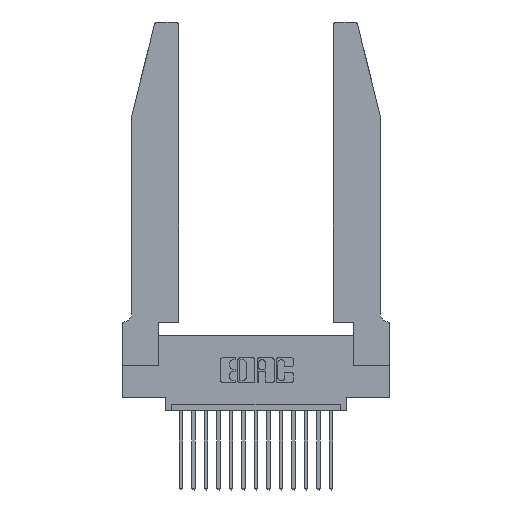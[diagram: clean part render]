
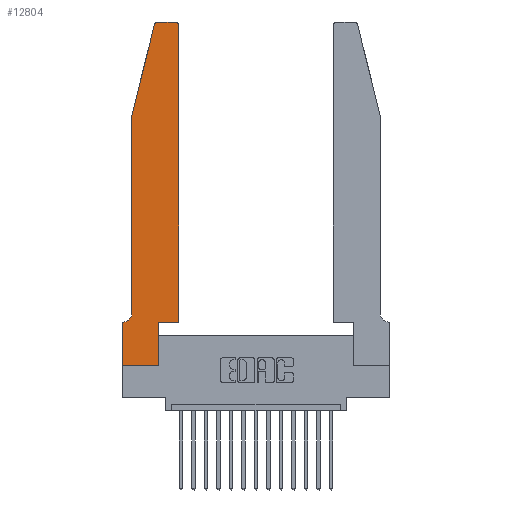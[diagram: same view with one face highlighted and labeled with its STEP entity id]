
A CAD part, top view. The second image highlights one B-rep face of the part: STEP entity #12804.
In plain terms, the highlighted planar face has unit normal (0, 0, 1).
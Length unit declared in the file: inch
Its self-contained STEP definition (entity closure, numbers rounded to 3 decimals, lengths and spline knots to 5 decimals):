
#98 = VECTOR ( 'NONE', #12148, 39.37008 ) ;
#214 = EDGE_CURVE ( 'NONE', #18326, #15537, #3929, .T. ) ;
#278 = VECTOR ( 'NONE', #9885, 39.37008 ) ;
#992 = CARTESIAN_POINT ( 'NONE',  ( 0.4505, 0.35, 0.37 ) ) ;
#1054 = VERTEX_POINT ( 'NONE', #13130 ) ;
#1116 = DIRECTION ( 'NONE',  ( 1., 0., 0. ) ) ;
#1184 = DIRECTION ( 'NONE',  ( 0., 0., -1. ) ) ;
#1329 = LINE ( 'NONE', #18397, #10377 ) ;
#1780 = ORIENTED_EDGE ( 'NONE', *, *, #1975, .T. ) ;
#1890 = AXIS2_PLACEMENT_3D ( 'NONE', #17011, #1184, #10670 ) ;
#1975 = EDGE_CURVE ( 'NONE', #15537, #5987, #3464, .T. ) ;
#1980 = DIRECTION ( 'NONE',  ( 1., 0., 0. ) ) ;
#1981 = VERTEX_POINT ( 'NONE', #3384 ) ;
#2617 = VERTEX_POINT ( 'NONE', #7955 ) ;
#2734 = EDGE_CURVE ( 'NONE', #1981, #7462, #11979, .T. ) ;
#3241 = CARTESIAN_POINT ( 'NONE',  ( 0.2605, 2.75, 0.37 ) ) ;
#3384 = CARTESIAN_POINT ( 'NONE',  ( 0.284, 2.75, 0.37 ) ) ;
#3448 = CARTESIAN_POINT ( 'NONE',  ( 0.2865, 0., 0.37 ) ) ;
#3463 = VERTEX_POINT ( 'NONE', #18270 ) ;
#3464 = LINE ( 'NONE', #7441, #11129 ) ;
#3508 = EDGE_LOOP ( 'NONE', ( #17701, #14174, #8043, #7591, #17520, #9115, #18115, #8007, #11388, #1780, #12761, #15362 ) ) ;
#3929 = LINE ( 'NONE', #10713, #98 ) ;
#4223 = DIRECTION ( 'NONE',  ( 1., 0., 0. ) ) ;
#4248 = VECTOR ( 'NONE', #13161, 39.37008 ) ;
#4614 = EDGE_CURVE ( 'NONE', #11953, #18326, #1329, .T. ) ;
#4631 = CARTESIAN_POINT ( 'NONE',  ( 0.0755, 2., 0.37 ) ) ;
#5124 = VECTOR ( 'NONE', #17776, 39.37008 ) ;
#5360 = CARTESIAN_POINT ( 'NONE',  ( 0.0755, 2., 0.37 ) ) ;
#5379 = DIRECTION ( 'NONE',  ( 0., 1., 0. ) ) ;
#5501 = DIRECTION ( 'NONE',  ( 0., 0., 1. ) ) ;
#5647 = CARTESIAN_POINT ( 'NONE',  ( 0.2865, 0.35, 0.37 ) ) ;
#5987 = VERTEX_POINT ( 'NONE', #14329 ) ;
#6363 = PLANE ( 'NONE',  #10347 ) ;
#6432 = CARTESIAN_POINT ( 'NONE',  ( 0., 0.35, 0.37 ) ) ;
#6682 = EDGE_CURVE ( 'NONE', #3463, #18084, #14528, .T. ) ;
#7014 = CARTESIAN_POINT ( 'NONE',  ( 0.284, 2.72, 0.37 ) ) ;
#7058 = LINE ( 'NONE', #7391, #278 ) ;
#7292 = AXIS2_PLACEMENT_3D ( 'NONE', #7014, #5501, #1116 ) ;
#7391 = CARTESIAN_POINT ( 'NONE',  ( 0., 0., 0.37 ) ) ;
#7441 = CARTESIAN_POINT ( 'NONE',  ( 0.4505, 0.35, 0.37 ) ) ;
#7462 = VERTEX_POINT ( 'NONE', #17816 ) ;
#7591 = ORIENTED_EDGE ( 'NONE', *, *, #6682, .T. ) ;
#7629 = VECTOR ( 'NONE', #16614, 39.37008 ) ;
#7668 = VECTOR ( 'NONE', #15334, 39.37008 ) ;
#7924 = DIRECTION ( 'NONE',  ( 0., 0., 1. ) ) ;
#7955 = CARTESIAN_POINT ( 'NONE',  ( 0.4205, 2.75, 0.37 ) ) ;
#8007 = ORIENTED_EDGE ( 'NONE', *, *, #4614, .T. ) ;
#8043 = ORIENTED_EDGE ( 'NONE', *, *, #12394, .T. ) ;
#8228 = DIRECTION ( 'NONE',  ( 1., 0., 0. ) ) ;
#8265 = EDGE_CURVE ( 'NONE', #5987, #18266, #18032, .T. ) ;
#8780 = LINE ( 'NONE', #10931, #7629 ) ;
#9115 = ORIENTED_EDGE ( 'NONE', *, *, #14319, .T. ) ;
#9436 = CARTESIAN_POINT ( 'NONE',  ( 0., 0.35, 0.37 ) ) ;
#9878 = AXIS2_PLACEMENT_3D ( 'NONE', #12778, #16868, #4223 ) ;
#9885 = DIRECTION ( 'NONE',  ( 0., -1., 0. ) ) ;
#9929 = EDGE_CURVE ( 'NONE', #17885, #11953, #7058, .T. ) ;
#10288 = VECTOR ( 'NONE', #5379, 39.37008 ) ;
#10347 = AXIS2_PLACEMENT_3D ( 'NONE', #9436, #7924, #17875 ) ;
#10377 = VECTOR ( 'NONE', #8228, 39.37008 ) ;
#10572 = LINE ( 'NONE', #5360, #7668 ) ;
#10670 = DIRECTION ( 'NONE',  ( -1., 0., 0. ) ) ;
#10713 = CARTESIAN_POINT ( 'NONE',  ( 0.2865, 0.35, 0.37 ) ) ;
#10931 = CARTESIAN_POINT ( 'NONE',  ( 0.0755, 0.35, 0.37 ) ) ;
#10985 = CIRCLE ( 'NONE', #1890, 0.07 ) ;
#11129 = VECTOR ( 'NONE', #1980, 39.37008 ) ;
#11312 = CARTESIAN_POINT ( 'NONE',  ( 0.4505, 2.72, 0.37 ) ) ;
#11388 = ORIENTED_EDGE ( 'NONE', *, *, #214, .T. ) ;
#11953 = VERTEX_POINT ( 'NONE', #17899 ) ;
#11979 = CIRCLE ( 'NONE', #7292, 0.03 ) ;
#12148 = DIRECTION ( 'NONE',  ( 0., 1., 0. ) ) ;
#12394 = EDGE_CURVE ( 'NONE', #7462, #3463, #10572, .T. ) ;
#12761 = ORIENTED_EDGE ( 'NONE', *, *, #8265, .T. ) ;
#12778 = CARTESIAN_POINT ( 'NONE',  ( 0.4205, 2.72, 0.37 ) ) ;
#12804 = ADVANCED_FACE ( 'NONE', ( #17467 ), #6363, .T. ) ;
#13130 = CARTESIAN_POINT ( 'NONE',  ( 0.0055, 0.35, 0.37 ) ) ;
#13161 = DIRECTION ( 'NONE',  ( -1., 0., 0. ) ) ;
#13432 = CIRCLE ( 'NONE', #9878, 0.03 ) ;
#14097 = EDGE_CURVE ( 'NONE', #18266, #2617, #13432, .T. ) ;
#14174 = ORIENTED_EDGE ( 'NONE', *, *, #2734, .T. ) ;
#14319 = EDGE_CURVE ( 'NONE', #1054, #17885, #8780, .T. ) ;
#14329 = CARTESIAN_POINT ( 'NONE',  ( 0.4505, 0.35, 0.37 ) ) ;
#14447 = EDGE_CURVE ( 'NONE', #18084, #1054, #10985, .T. ) ;
#14528 = LINE ( 'NONE', #4631, #5124 ) ;
#14764 = EDGE_CURVE ( 'NONE', #2617, #1981, #16724, .T. ) ;
#15334 = DIRECTION ( 'NONE',  ( -0.239, -0.971, 0. ) ) ;
#15362 = ORIENTED_EDGE ( 'NONE', *, *, #14097, .T. ) ;
#15537 = VERTEX_POINT ( 'NONE', #5647 ) ;
#15803 = CARTESIAN_POINT ( 'NONE',  ( 0.0755, 0.42, 0.37 ) ) ;
#16614 = DIRECTION ( 'NONE',  ( -1., 0., 0. ) ) ;
#16724 = LINE ( 'NONE', #3241, #4248 ) ;
#16868 = DIRECTION ( 'NONE',  ( 0., 0., 1. ) ) ;
#17011 = CARTESIAN_POINT ( 'NONE',  ( 0.0055, 0.42, 0.37 ) ) ;
#17467 = FACE_OUTER_BOUND ( 'NONE', #3508, .T. ) ;
#17520 = ORIENTED_EDGE ( 'NONE', *, *, #14447, .T. ) ;
#17701 = ORIENTED_EDGE ( 'NONE', *, *, #14764, .T. ) ;
#17776 = DIRECTION ( 'NONE',  ( 0., -1., 0. ) ) ;
#17816 = CARTESIAN_POINT ( 'NONE',  ( 0.25487, 2.72718, 0.37 ) ) ;
#17875 = DIRECTION ( 'NONE',  ( 1., 0., 0. ) ) ;
#17885 = VERTEX_POINT ( 'NONE', #6432 ) ;
#17899 = CARTESIAN_POINT ( 'NONE',  ( 0., 0., 0.37 ) ) ;
#18032 = LINE ( 'NONE', #992, #10288 ) ;
#18084 = VERTEX_POINT ( 'NONE', #15803 ) ;
#18115 = ORIENTED_EDGE ( 'NONE', *, *, #9929, .T. ) ;
#18266 = VERTEX_POINT ( 'NONE', #11312 ) ;
#18270 = CARTESIAN_POINT ( 'NONE',  ( 0.0755, 2., 0.37 ) ) ;
#18326 = VERTEX_POINT ( 'NONE', #3448 ) ;
#18397 = CARTESIAN_POINT ( 'NONE',  ( 0., 0., 0.37 ) ) ;
